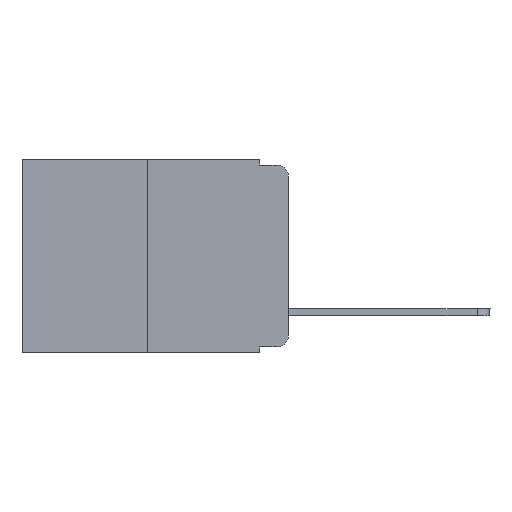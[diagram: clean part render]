
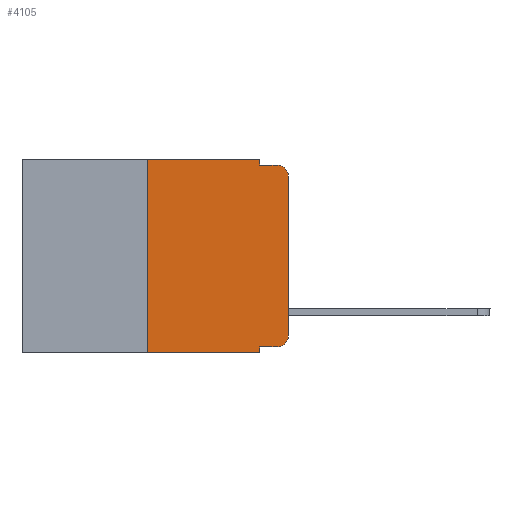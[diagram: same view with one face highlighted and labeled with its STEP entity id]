
A CAD part, left-side view. The second image highlights one B-rep face of the part: STEP entity #4105.
In plain terms, the highlighted planar face has unit normal (-1, 0, 0).
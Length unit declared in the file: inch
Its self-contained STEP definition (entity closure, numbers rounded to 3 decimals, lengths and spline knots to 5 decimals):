
#184 = CARTESIAN_POINT ( 'NONE',  ( 0., 0.02, -0.03 ) ) ;
#197 = VECTOR ( 'NONE', #4160, 39.37008 ) ;
#239 = LINE ( 'NONE', #1866, #5392 ) ;
#274 = ORIENTED_EDGE ( 'NONE', *, *, #6869, .F. ) ;
#379 = EDGE_CURVE ( 'NONE', #7449, #10427, #1560, .T. ) ;
#412 = ORIENTED_EDGE ( 'NONE', *, *, #8443, .F. ) ;
#749 = LINE ( 'NONE', #6465, #9796 ) ;
#792 = ORIENTED_EDGE ( 'NONE', *, *, #7330, .T. ) ;
#824 = CARTESIAN_POINT ( 'NONE',  ( 0., 0.02, -0.01 ) ) ;
#829 = AXIS2_PLACEMENT_3D ( 'NONE', #8510, #7433, #5265 ) ;
#1136 = CARTESIAN_POINT ( 'NONE',  ( 0., 0., -0.313 ) ) ;
#1326 = FACE_OUTER_BOUND ( 'NONE', #3850, .T. ) ;
#1560 = LINE ( 'NONE', #6522, #197 ) ;
#1696 = EDGE_CURVE ( 'NONE', #10427, #2731, #10680, .T. ) ;
#1866 = CARTESIAN_POINT ( 'NONE',  ( 0., 0.473, -0.343 ) ) ;
#2087 = CARTESIAN_POINT ( 'NONE',  ( 0., 0.051, -0.01 ) ) ;
#2318 = CARTESIAN_POINT ( 'NONE',  ( 0., 0.051, 0. ) ) ;
#2731 = VERTEX_POINT ( 'NONE', #1136 ) ;
#2910 = CARTESIAN_POINT ( 'NONE',  ( 0., 0.473, 0. ) ) ;
#2946 = EDGE_CURVE ( 'NONE', #4371, #10618, #10625, .T. ) ;
#3105 = VERTEX_POINT ( 'NONE', #6121 ) ;
#3206 = CARTESIAN_POINT ( 'NONE',  ( 0., 0.473, 0. ) ) ;
#3473 = DIRECTION ( 'NONE',  ( 0., -1., 0. ) ) ;
#3538 = VECTOR ( 'NONE', #8645, 39.37008 ) ;
#3559 = AXIS2_PLACEMENT_3D ( 'NONE', #2910, #5439, #7985 ) ;
#3727 = EDGE_CURVE ( 'NONE', #7449, #7139, #10430, .T. ) ;
#3850 = EDGE_LOOP ( 'NONE', ( #9359, #792, #10550, #412, #7523, #274, #10346, #5880, #6363, #7367 ) ) ;
#4105 = ADVANCED_FACE ( 'NONE', ( #1326 ), #7150, .F. ) ;
#4136 = VERTEX_POINT ( 'NONE', #2087 ) ;
#4160 = DIRECTION ( 'NONE',  ( 0., -1., 0. ) ) ;
#4371 = VERTEX_POINT ( 'NONE', #8407 ) ;
#4551 = EDGE_CURVE ( 'NONE', #2731, #10619, #4664, .T. ) ;
#4664 = LINE ( 'NONE', #5325, #4775 ) ;
#4775 = VECTOR ( 'NONE', #10455, 39.37008 ) ;
#4987 = VECTOR ( 'NONE', #9826, 39.37008 ) ;
#5265 = DIRECTION ( 'NONE',  ( 0., 0., -1. ) ) ;
#5325 = CARTESIAN_POINT ( 'NONE',  ( 0., 0., 0. ) ) ;
#5392 = VECTOR ( 'NONE', #9238, 39.37008 ) ;
#5439 = DIRECTION ( 'NONE',  ( 1., 0., 0. ) ) ;
#5528 = CARTESIAN_POINT ( 'NONE',  ( 0., 0.051, -0.333 ) ) ;
#5727 = EDGE_CURVE ( 'NONE', #3105, #7139, #239, .T. ) ;
#5812 = DIRECTION ( 'NONE',  ( -1., 0., 0. ) ) ;
#5880 = ORIENTED_EDGE ( 'NONE', *, *, #3727, .F. ) ;
#5908 = LINE ( 'NONE', #9228, #6655 ) ;
#5927 = VERTEX_POINT ( 'NONE', #824 ) ;
#5986 = CIRCLE ( 'NONE', #6490, 0.02 ) ;
#6067 = EDGE_CURVE ( 'NONE', #4136, #5927, #10199, .T. ) ;
#6121 = CARTESIAN_POINT ( 'NONE',  ( 0., 0.25, -0.343 ) ) ;
#6252 = CARTESIAN_POINT ( 'NONE',  ( 0., 0., -0.03 ) ) ;
#6363 = ORIENTED_EDGE ( 'NONE', *, *, #379, .T. ) ;
#6465 = CARTESIAN_POINT ( 'NONE',  ( 0., 0.25, 0. ) ) ;
#6490 = AXIS2_PLACEMENT_3D ( 'NONE', #184, #5812, #7481 ) ;
#6522 = CARTESIAN_POINT ( 'NONE',  ( 0., 0.051, -0.333 ) ) ;
#6655 = VECTOR ( 'NONE', #8714, 39.37008 ) ;
#6869 = EDGE_CURVE ( 'NONE', #3105, #4371, #749, .T. ) ;
#7139 = VERTEX_POINT ( 'NONE', #9839 ) ;
#7150 = PLANE ( 'NONE',  #3559 ) ;
#7330 = EDGE_CURVE ( 'NONE', #10619, #5927, #5986, .T. ) ;
#7367 = ORIENTED_EDGE ( 'NONE', *, *, #1696, .T. ) ;
#7433 = DIRECTION ( 'NONE',  ( -1., 0., 0. ) ) ;
#7449 = VERTEX_POINT ( 'NONE', #5528 ) ;
#7481 = DIRECTION ( 'NONE',  ( 0., 0., -1. ) ) ;
#7523 = ORIENTED_EDGE ( 'NONE', *, *, #2946, .F. ) ;
#7985 = DIRECTION ( 'NONE',  ( 0., 0., -1. ) ) ;
#7998 = DIRECTION ( 'NONE',  ( 0., 0., 1. ) ) ;
#8166 = CARTESIAN_POINT ( 'NONE',  ( 0., 0.02, -0.333 ) ) ;
#8350 = CARTESIAN_POINT ( 'NONE',  ( 0., 0.051, -0.01 ) ) ;
#8407 = CARTESIAN_POINT ( 'NONE',  ( 0., 0.25, 0. ) ) ;
#8443 = EDGE_CURVE ( 'NONE', #10618, #4136, #5908, .T. ) ;
#8510 = CARTESIAN_POINT ( 'NONE',  ( 0., 0.02, -0.313 ) ) ;
#8645 = DIRECTION ( 'NONE',  ( 0., 0., -1. ) ) ;
#8714 = DIRECTION ( 'NONE',  ( 0., 0., -1. ) ) ;
#9228 = CARTESIAN_POINT ( 'NONE',  ( 0., 0.051, 0. ) ) ;
#9238 = DIRECTION ( 'NONE',  ( 0., -1., 0. ) ) ;
#9359 = ORIENTED_EDGE ( 'NONE', *, *, #4551, .T. ) ;
#9469 = CARTESIAN_POINT ( 'NONE',  ( 0., 0.051, 0. ) ) ;
#9557 = VECTOR ( 'NONE', #3473, 39.37008 ) ;
#9796 = VECTOR ( 'NONE', #7998, 39.37008 ) ;
#9826 = DIRECTION ( 'NONE',  ( 0., -1., 0. ) ) ;
#9839 = CARTESIAN_POINT ( 'NONE',  ( 0., 0.051, -0.343 ) ) ;
#10199 = LINE ( 'NONE', #8350, #9557 ) ;
#10346 = ORIENTED_EDGE ( 'NONE', *, *, #5727, .T. ) ;
#10427 = VERTEX_POINT ( 'NONE', #8166 ) ;
#10430 = LINE ( 'NONE', #2318, #3538 ) ;
#10455 = DIRECTION ( 'NONE',  ( 0., 0., 1. ) ) ;
#10550 = ORIENTED_EDGE ( 'NONE', *, *, #6067, .F. ) ;
#10618 = VERTEX_POINT ( 'NONE', #9469 ) ;
#10619 = VERTEX_POINT ( 'NONE', #6252 ) ;
#10625 = LINE ( 'NONE', #3206, #4987 ) ;
#10680 = CIRCLE ( 'NONE', #829, 0.02 ) ;
